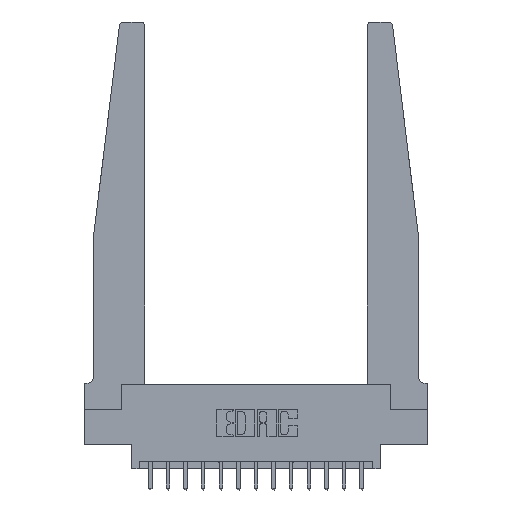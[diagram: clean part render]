
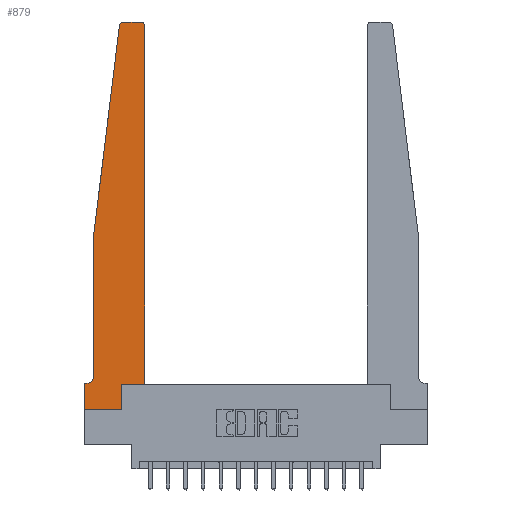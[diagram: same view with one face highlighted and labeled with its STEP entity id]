
A CAD part, top view. The second image highlights one B-rep face of the part: STEP entity #879.
In plain terms, the highlighted planar face has unit normal (0, 0, 1).
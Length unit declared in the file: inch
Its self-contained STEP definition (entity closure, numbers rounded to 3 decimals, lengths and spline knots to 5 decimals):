
#580 = CARTESIAN_POINT ( 'NONE',  ( 0.425, 0.18, 0.37 ) ) ;
#719 = CARTESIAN_POINT ( 'NONE',  ( 0., 0., 0.37 ) ) ;
#790 = LINE ( 'NONE', #4845, #1471 ) ;
#879 = ADVANCED_FACE ( 'NONE', ( #16980 ), #11581, .T. ) ;
#1095 = ORIENTED_EDGE ( 'NONE', *, *, #8095, .T. ) ;
#1208 = LINE ( 'NONE', #5341, #1790 ) ;
#1251 = CARTESIAN_POINT ( 'NONE',  ( 0.065, 0.2375, 0.37 ) ) ;
#1471 = VECTOR ( 'NONE', #17123, 39.37008 ) ;
#1631 = LINE ( 'NONE', #6978, #9740 ) ;
#1760 = DIRECTION ( 'NONE',  ( -1., 0., 0. ) ) ;
#1790 = VECTOR ( 'NONE', #12137, 39.37008 ) ;
#2373 = CARTESIAN_POINT ( 'NONE',  ( 0.065, 1.25, 0.37 ) ) ;
#2482 = CARTESIAN_POINT ( 'NONE',  ( 0.2605, 0.18, 0.37 ) ) ;
#2668 = EDGE_CURVE ( 'NONE', #11462, #5857, #16434, .T. ) ;
#2725 = CIRCLE ( 'NONE', #8187, 0.03 ) ;
#2910 = CARTESIAN_POINT ( 'NONE',  ( 0., 0.1875, 0.37 ) ) ;
#3168 = DIRECTION ( 'NONE',  ( 1., 0., 0. ) ) ;
#4185 = CARTESIAN_POINT ( 'NONE',  ( 0.065, 1.25, 0.37 ) ) ;
#4491 = VECTOR ( 'NONE', #13634, 39.37008 ) ;
#4685 = CARTESIAN_POINT ( 'NONE',  ( 0.2605, 0., 0.37 ) ) ;
#4730 = DIRECTION ( 'NONE',  ( -1., 0., 0. ) ) ;
#4845 = CARTESIAN_POINT ( 'NONE',  ( 0.425, 0.18, 0.37 ) ) ;
#4862 = ORIENTED_EDGE ( 'NONE', *, *, #2668, .T. ) ;
#5047 = VERTEX_POINT ( 'NONE', #14448 ) ;
#5139 = ORIENTED_EDGE ( 'NONE', *, *, #8681, .T. ) ;
#5198 = VERTEX_POINT ( 'NONE', #580 ) ;
#5279 = ORIENTED_EDGE ( 'NONE', *, *, #5651, .T. ) ;
#5341 = CARTESIAN_POINT ( 'NONE',  ( 0.065, 0.1875, 0.37 ) ) ;
#5388 = ORIENTED_EDGE ( 'NONE', *, *, #6974, .T. ) ;
#5399 = ORIENTED_EDGE ( 'NONE', *, *, #15317, .T. ) ;
#5651 = EDGE_CURVE ( 'NONE', #14740, #6768, #10961, .T. ) ;
#5802 = CARTESIAN_POINT ( 'NONE',  ( 0.065, 1.25, 0.37 ) ) ;
#5826 = CARTESIAN_POINT ( 'NONE',  ( 0.015, 0.2375, 0.37 ) ) ;
#5857 = VERTEX_POINT ( 'NONE', #14596 ) ;
#6297 = CARTESIAN_POINT ( 'NONE',  ( 0.25, 2.75, 0.37 ) ) ;
#6590 = VECTOR ( 'NONE', #8271, 39.37008 ) ;
#6669 = ORIENTED_EDGE ( 'NONE', *, *, #16361, .T. ) ;
#6768 = VERTEX_POINT ( 'NONE', #2482 ) ;
#6974 = EDGE_CURVE ( 'NONE', #5857, #10041, #8909, .T. ) ;
#6978 = CARTESIAN_POINT ( 'NONE',  ( 0.425, 0.18, 0.37 ) ) ;
#7578 = CARTESIAN_POINT ( 'NONE',  ( 0., 0.1875, 0.37 ) ) ;
#7832 = EDGE_CURVE ( 'NONE', #5198, #15422, #1631, .T. ) ;
#7856 = CARTESIAN_POINT ( 'NONE',  ( 0.425, 2.72, 0.37 ) ) ;
#8095 = EDGE_CURVE ( 'NONE', #15422, #17110, #2725, .T. ) ;
#8187 = AXIS2_PLACEMENT_3D ( 'NONE', #14093, #17330, #14951 ) ;
#8271 = DIRECTION ( 'NONE',  ( 0., 1., 0. ) ) ;
#8622 = DIRECTION ( 'NONE',  ( -0.122, -0.992, 0. ) ) ;
#8681 = EDGE_CURVE ( 'NONE', #5047, #14740, #11061, .T. ) ;
#8780 = DIRECTION ( 'NONE',  ( 0., 0., -1. ) ) ;
#8909 = LINE ( 'NONE', #4185, #15646 ) ;
#8984 = CARTESIAN_POINT ( 'NONE',  ( 0.395, 2.75, 0.37 ) ) ;
#9318 = DIRECTION ( 'NONE',  ( 0., -1., 0. ) ) ;
#9550 = DIRECTION ( 'NONE',  ( 0., 1., 0. ) ) ;
#9573 = LINE ( 'NONE', #2373, #14198 ) ;
#9590 = EDGE_LOOP ( 'NONE', ( #10714, #4862, #5388, #16689, #5399, #16159, #6669, #5139, #5279, #14466, #15798, #1095 ) ) ;
#9674 = VECTOR ( 'NONE', #4730, 39.37008 ) ;
#9740 = VECTOR ( 'NONE', #9550, 39.37008 ) ;
#10029 = VERTEX_POINT ( 'NONE', #2910 ) ;
#10041 = VERTEX_POINT ( 'NONE', #5802 ) ;
#10228 = DIRECTION ( 'NONE',  ( 0., 0., 1. ) ) ;
#10251 = DIRECTION ( 'NONE',  ( 0., 0., 1. ) ) ;
#10427 = EDGE_CURVE ( 'NONE', #6768, #5198, #790, .T. ) ;
#10490 = VERTEX_POINT ( 'NONE', #17302 ) ;
#10714 = ORIENTED_EDGE ( 'NONE', *, *, #17101, .T. ) ;
#10961 = LINE ( 'NONE', #15236, #6590 ) ;
#11061 = LINE ( 'NONE', #16502, #4491 ) ;
#11369 = VECTOR ( 'NONE', #11493, 39.37008 ) ;
#11440 = AXIS2_PLACEMENT_3D ( 'NONE', #7578, #10251, #3168 ) ;
#11462 = VERTEX_POINT ( 'NONE', #15435 ) ;
#11493 = DIRECTION ( 'NONE',  ( 0., -1., 0. ) ) ;
#11565 = CARTESIAN_POINT ( 'NONE',  ( 0.27653, 2.72, 0.37 ) ) ;
#11581 = PLANE ( 'NONE',  #11440 ) ;
#11656 = AXIS2_PLACEMENT_3D ( 'NONE', #5826, #8780, #1760 ) ;
#12137 = DIRECTION ( 'NONE',  ( -1., 0., 0. ) ) ;
#12693 = EDGE_CURVE ( 'NONE', #10041, #16894, #9573, .T. ) ;
#12981 = LINE ( 'NONE', #6297, #9674 ) ;
#13570 = AXIS2_PLACEMENT_3D ( 'NONE', #11565, #10228, #15692 ) ;
#13634 = DIRECTION ( 'NONE',  ( 1., 0., 0. ) ) ;
#14093 = CARTESIAN_POINT ( 'NONE',  ( 0.395, 2.72, 0.37 ) ) ;
#14198 = VECTOR ( 'NONE', #9318, 39.37008 ) ;
#14340 = EDGE_CURVE ( 'NONE', #10490, #10029, #1208, .T. ) ;
#14448 = CARTESIAN_POINT ( 'NONE',  ( 0., 0., 0.37 ) ) ;
#14466 = ORIENTED_EDGE ( 'NONE', *, *, #10427, .T. ) ;
#14596 = CARTESIAN_POINT ( 'NONE',  ( 0.24675, 2.72367, 0.37 ) ) ;
#14740 = VERTEX_POINT ( 'NONE', #4685 ) ;
#14951 = DIRECTION ( 'NONE',  ( 1., 0., 0. ) ) ;
#15236 = CARTESIAN_POINT ( 'NONE',  ( 0.2605, 0.18, 0.37 ) ) ;
#15317 = EDGE_CURVE ( 'NONE', #16894, #10490, #15680, .T. ) ;
#15422 = VERTEX_POINT ( 'NONE', #7856 ) ;
#15435 = CARTESIAN_POINT ( 'NONE',  ( 0.27653, 2.75, 0.37 ) ) ;
#15646 = VECTOR ( 'NONE', #8622, 39.37008 ) ;
#15680 = CIRCLE ( 'NONE', #11656, 0.05 ) ;
#15692 = DIRECTION ( 'NONE',  ( 1., 0., 0. ) ) ;
#15798 = ORIENTED_EDGE ( 'NONE', *, *, #7832, .T. ) ;
#16159 = ORIENTED_EDGE ( 'NONE', *, *, #14340, .T. ) ;
#16361 = EDGE_CURVE ( 'NONE', #10029, #5047, #17237, .T. ) ;
#16434 = CIRCLE ( 'NONE', #13570, 0.03 ) ;
#16502 = CARTESIAN_POINT ( 'NONE',  ( 0., 0., 0.37 ) ) ;
#16689 = ORIENTED_EDGE ( 'NONE', *, *, #12693, .T. ) ;
#16894 = VERTEX_POINT ( 'NONE', #1251 ) ;
#16980 = FACE_OUTER_BOUND ( 'NONE', #9590, .T. ) ;
#17101 = EDGE_CURVE ( 'NONE', #17110, #11462, #12981, .T. ) ;
#17110 = VERTEX_POINT ( 'NONE', #8984 ) ;
#17123 = DIRECTION ( 'NONE',  ( 1., 0., 0. ) ) ;
#17237 = LINE ( 'NONE', #719, #11369 ) ;
#17302 = CARTESIAN_POINT ( 'NONE',  ( 0.015, 0.1875, 0.37 ) ) ;
#17330 = DIRECTION ( 'NONE',  ( 0., 0., 1. ) ) ;
